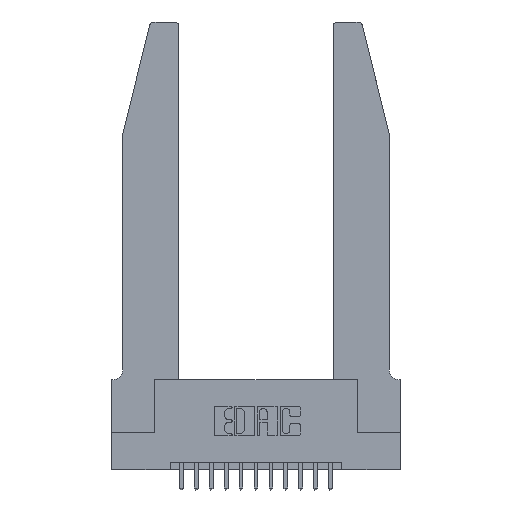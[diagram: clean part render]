
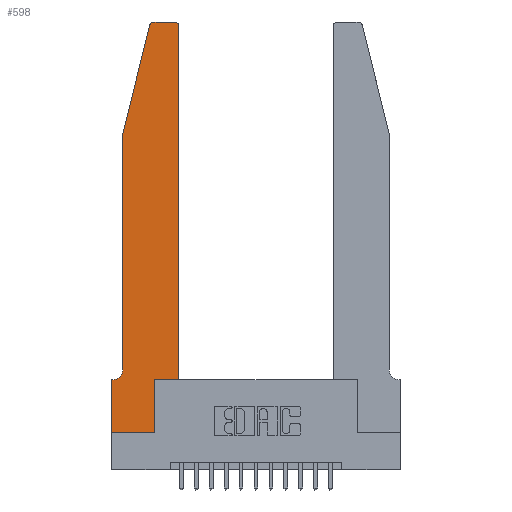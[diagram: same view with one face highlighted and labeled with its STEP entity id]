
A CAD part, top view. The second image highlights one B-rep face of the part: STEP entity #598.
In plain terms, the highlighted planar face has unit normal (0, 0, 1).
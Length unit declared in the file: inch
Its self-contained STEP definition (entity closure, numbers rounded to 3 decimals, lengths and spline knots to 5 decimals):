
#104 = AXIS2_PLACEMENT_3D ( 'NONE', #14632, #249, #910 ) ;
#151 = VERTEX_POINT ( 'NONE', #7603 ) ;
#164 = CIRCLE ( 'NONE', #104, 0.03 ) ;
#167 = EDGE_CURVE ( 'NONE', #11001, #4482, #4206, .T. ) ;
#249 = DIRECTION ( 'NONE',  ( 0., 0., 1. ) ) ;
#295 = EDGE_CURVE ( 'NONE', #13856, #11001, #1206, .T. ) ;
#354 = EDGE_CURVE ( 'NONE', #12415, #3944, #14656, .T. ) ;
#396 = CARTESIAN_POINT ( 'NONE',  ( 0.2865, 0.35, 0.37 ) ) ;
#598 = ADVANCED_FACE ( 'NONE', ( #13973 ), #6932, .T. ) ;
#784 = CARTESIAN_POINT ( 'NONE',  ( 0.2865, 0.35, 0.37 ) ) ;
#910 = DIRECTION ( 'NONE',  ( 1., 0., 0. ) ) ;
#957 = ORIENTED_EDGE ( 'NONE', *, *, #2264, .T. ) ;
#1101 = ORIENTED_EDGE ( 'NONE', *, *, #9592, .T. ) ;
#1206 = LINE ( 'NONE', #6678, #4413 ) ;
#1447 = CARTESIAN_POINT ( 'NONE',  ( 0., 0., 0.37 ) ) ;
#2190 = LINE ( 'NONE', #1447, #11794 ) ;
#2264 = EDGE_CURVE ( 'NONE', #4482, #151, #15261, .T. ) ;
#2533 = ORIENTED_EDGE ( 'NONE', *, *, #295, .T. ) ;
#2604 = CARTESIAN_POINT ( 'NONE',  ( 0.4505, 0.35, 0.37 ) ) ;
#2699 = VERTEX_POINT ( 'NONE', #5062 ) ;
#2934 = EDGE_CURVE ( 'NONE', #3944, #13856, #8161, .T. ) ;
#2958 = EDGE_LOOP ( 'NONE', ( #6802, #1101, #17290, #8596, #16020, #4789, #11266, #7703, #8132, #2533, #7722, #957 ) ) ;
#3336 = VECTOR ( 'NONE', #6816, 39.37008 ) ;
#3685 = VERTEX_POINT ( 'NONE', #4581 ) ;
#3727 = CARTESIAN_POINT ( 'NONE',  ( 0.284, 2.75, 0.37 ) ) ;
#3814 = CARTESIAN_POINT ( 'NONE',  ( 0., 0.35, 0.37 ) ) ;
#3828 = DIRECTION ( 'NONE',  ( 0., 1., 0. ) ) ;
#3944 = VERTEX_POINT ( 'NONE', #7929 ) ;
#4089 = DIRECTION ( 'NONE',  ( 1., 0., 0. ) ) ;
#4154 = CARTESIAN_POINT ( 'NONE',  ( 0.4205, 2.72, 0.37 ) ) ;
#4206 = LINE ( 'NONE', #7877, #12280 ) ;
#4351 = DIRECTION ( 'NONE',  ( 1., 0., 0. ) ) ;
#4355 = LINE ( 'NONE', #11241, #11582 ) ;
#4377 = EDGE_CURVE ( 'NONE', #3685, #4946, #12129, .T. ) ;
#4413 = VECTOR ( 'NONE', #4089, 39.37008 ) ;
#4482 = VERTEX_POINT ( 'NONE', #12715 ) ;
#4485 = DIRECTION ( 'NONE',  ( -0.239, -0.971, 0. ) ) ;
#4581 = CARTESIAN_POINT ( 'NONE',  ( 0.0755, 0.42, 0.37 ) ) ;
#4789 = ORIENTED_EDGE ( 'NONE', *, *, #16258, .T. ) ;
#4946 = VERTEX_POINT ( 'NONE', #9897 ) ;
#5062 = CARTESIAN_POINT ( 'NONE',  ( 0.0755, 2., 0.37 ) ) ;
#5577 = CARTESIAN_POINT ( 'NONE',  ( 0., 0., 0.37 ) ) ;
#5780 = AXIS2_PLACEMENT_3D ( 'NONE', #9066, #17031, #11804 ) ;
#5850 = VERTEX_POINT ( 'NONE', #3727 ) ;
#6678 = CARTESIAN_POINT ( 'NONE',  ( 0.4505, 0.35, 0.37 ) ) ;
#6802 = ORIENTED_EDGE ( 'NONE', *, *, #8513, .T. ) ;
#6816 = DIRECTION ( 'NONE',  ( 1., 0., 0. ) ) ;
#6817 = VERTEX_POINT ( 'NONE', #9953 ) ;
#6932 = PLANE ( 'NONE',  #14624 ) ;
#7603 = CARTESIAN_POINT ( 'NONE',  ( 0.4205, 2.75, 0.37 ) ) ;
#7703 = ORIENTED_EDGE ( 'NONE', *, *, #354, .T. ) ;
#7722 = ORIENTED_EDGE ( 'NONE', *, *, #167, .T. ) ;
#7782 = DIRECTION ( 'NONE',  ( -1., 0., 0. ) ) ;
#7877 = CARTESIAN_POINT ( 'NONE',  ( 0.4505, 0.35, 0.37 ) ) ;
#7929 = CARTESIAN_POINT ( 'NONE',  ( 0.2865, 0., 0.37 ) ) ;
#8082 = EDGE_CURVE ( 'NONE', #2699, #3685, #12467, .T. ) ;
#8132 = ORIENTED_EDGE ( 'NONE', *, *, #2934, .T. ) ;
#8161 = LINE ( 'NONE', #784, #14332 ) ;
#8316 = DIRECTION ( 'NONE',  ( 0., 0., 1. ) ) ;
#8513 = EDGE_CURVE ( 'NONE', #151, #5850, #11151, .T. ) ;
#8596 = ORIENTED_EDGE ( 'NONE', *, *, #8082, .T. ) ;
#8599 = CARTESIAN_POINT ( 'NONE',  ( 0., 0.35, 0.37 ) ) ;
#9066 = CARTESIAN_POINT ( 'NONE',  ( 0.0055, 0.42, 0.37 ) ) ;
#9273 = DIRECTION ( 'NONE',  ( 0., -1., 0. ) ) ;
#9390 = CARTESIAN_POINT ( 'NONE',  ( 0.0755, 2., 0.37 ) ) ;
#9592 = EDGE_CURVE ( 'NONE', #5850, #6817, #164, .T. ) ;
#9654 = EDGE_CURVE ( 'NONE', #16567, #12415, #2190, .T. ) ;
#9897 = CARTESIAN_POINT ( 'NONE',  ( 0.0055, 0.35, 0.37 ) ) ;
#9953 = CARTESIAN_POINT ( 'NONE',  ( 0.25487, 2.72718, 0.37 ) ) ;
#11001 = VERTEX_POINT ( 'NONE', #2604 ) ;
#11093 = DIRECTION ( 'NONE',  ( 0., 0., 1. ) ) ;
#11144 = DIRECTION ( 'NONE',  ( 0., -1., 0. ) ) ;
#11151 = LINE ( 'NONE', #14369, #12018 ) ;
#11241 = CARTESIAN_POINT ( 'NONE',  ( 0.0755, 2., 0.37 ) ) ;
#11266 = ORIENTED_EDGE ( 'NONE', *, *, #9654, .T. ) ;
#11489 = CARTESIAN_POINT ( 'NONE',  ( 0.0755, 0.35, 0.37 ) ) ;
#11582 = VECTOR ( 'NONE', #4485, 39.37008 ) ;
#11794 = VECTOR ( 'NONE', #11144, 39.37008 ) ;
#11804 = DIRECTION ( 'NONE',  ( -1., 0., 0. ) ) ;
#11887 = AXIS2_PLACEMENT_3D ( 'NONE', #4154, #8316, #12246 ) ;
#12018 = VECTOR ( 'NONE', #7782, 39.37008 ) ;
#12129 = CIRCLE ( 'NONE', #5780, 0.07 ) ;
#12246 = DIRECTION ( 'NONE',  ( 1., 0., 0. ) ) ;
#12280 = VECTOR ( 'NONE', #3828, 39.37008 ) ;
#12415 = VERTEX_POINT ( 'NONE', #14199 ) ;
#12467 = LINE ( 'NONE', #9390, #17552 ) ;
#12715 = CARTESIAN_POINT ( 'NONE',  ( 0.4505, 2.72, 0.37 ) ) ;
#12968 = DIRECTION ( 'NONE',  ( -1., 0., 0. ) ) ;
#13856 = VERTEX_POINT ( 'NONE', #396 ) ;
#13973 = FACE_OUTER_BOUND ( 'NONE', #2958, .T. ) ;
#14199 = CARTESIAN_POINT ( 'NONE',  ( 0., 0., 0.37 ) ) ;
#14332 = VECTOR ( 'NONE', #15679, 39.37008 ) ;
#14369 = CARTESIAN_POINT ( 'NONE',  ( 0.2605, 2.75, 0.37 ) ) ;
#14479 = EDGE_CURVE ( 'NONE', #6817, #2699, #4355, .T. ) ;
#14624 = AXIS2_PLACEMENT_3D ( 'NONE', #8599, #11093, #4351 ) ;
#14632 = CARTESIAN_POINT ( 'NONE',  ( 0.284, 2.72, 0.37 ) ) ;
#14656 = LINE ( 'NONE', #5577, #3336 ) ;
#15261 = CIRCLE ( 'NONE', #11887, 0.03 ) ;
#15679 = DIRECTION ( 'NONE',  ( 0., 1., 0. ) ) ;
#16020 = ORIENTED_EDGE ( 'NONE', *, *, #4377, .T. ) ;
#16258 = EDGE_CURVE ( 'NONE', #4946, #16567, #16807, .T. ) ;
#16567 = VERTEX_POINT ( 'NONE', #3814 ) ;
#16807 = LINE ( 'NONE', #11489, #17449 ) ;
#17031 = DIRECTION ( 'NONE',  ( 0., 0., -1. ) ) ;
#17290 = ORIENTED_EDGE ( 'NONE', *, *, #14479, .T. ) ;
#17449 = VECTOR ( 'NONE', #12968, 39.37008 ) ;
#17552 = VECTOR ( 'NONE', #9273, 39.37008 ) ;
